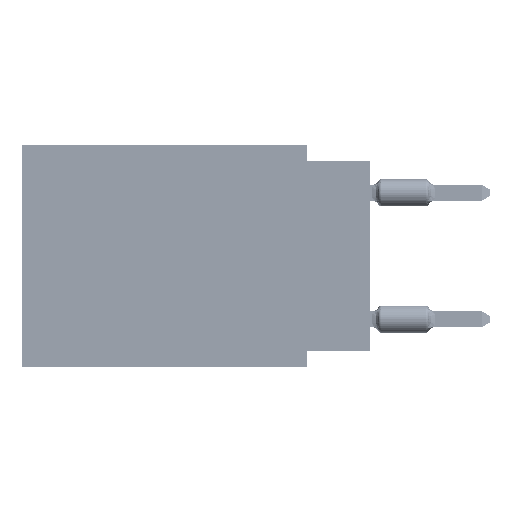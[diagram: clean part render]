
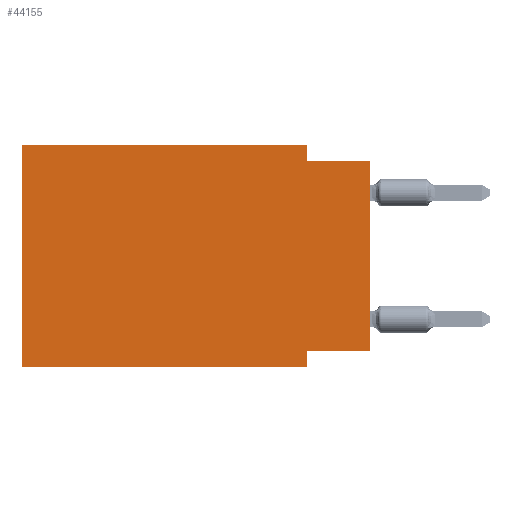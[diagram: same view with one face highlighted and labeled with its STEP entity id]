
A CAD part, left-side view. The second image highlights one B-rep face of the part: STEP entity #44155.
In plain terms, the highlighted planar face has unit normal (-1, 0, 0).
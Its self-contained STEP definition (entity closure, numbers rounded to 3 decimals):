
#339 = DIRECTION ( 'NONE',  ( 0., 0., 1. ) ) ;
#1045 = VECTOR ( 'NONE', #78806, 1000. ) ;
#1608 = CARTESIAN_POINT ( 'NONE',  ( 0., 0., -0.635 ) ) ;
#4545 = EDGE_CURVE ( 'NONE', #62421, #34760, #31598, .T. ) ;
#9363 = VERTEX_POINT ( 'NONE', #24462 ) ;
#10280 = CARTESIAN_POINT ( 'NONE',  ( 0., 13.97, 0. ) ) ;
#11450 = CARTESIAN_POINT ( 'NONE',  ( 0., 2.54, -8.255 ) ) ;
#14645 = EDGE_CURVE ( 'NONE', #9363, #31797, #24974, .T. ) ;
#15021 = CARTESIAN_POINT ( 'NONE',  ( 0., 0., 0. ) ) ;
#16466 = DIRECTION ( 'NONE',  ( 0., 0., -1. ) ) ;
#16555 = DIRECTION ( 'NONE',  ( 0., 0., -1. ) ) ;
#16689 = VECTOR ( 'NONE', #16466, 1000. ) ;
#17464 = PLANE ( 'NONE',  #34880 ) ;
#17490 = VERTEX_POINT ( 'NONE', #1608 ) ;
#18042 = LINE ( 'NONE', #81406, #1045 ) ;
#20534 = ORIENTED_EDGE ( 'NONE', *, *, #48890, .T. ) ;
#22259 = LINE ( 'NONE', #86538, #33979 ) ;
#22515 = LINE ( 'NONE', #44086, #33355 ) ;
#23358 = CARTESIAN_POINT ( 'NONE',  ( 0., 2.54, 0. ) ) ;
#23904 = FACE_OUTER_BOUND ( 'NONE', #74690, .T. ) ;
#24462 = CARTESIAN_POINT ( 'NONE',  ( 0., 13.97, -8.89 ) ) ;
#24974 = LINE ( 'NONE', #10280, #47477 ) ;
#25876 = DIRECTION ( 'NONE',  ( 0., 0., 1. ) ) ;
#25960 = EDGE_CURVE ( 'NONE', #31797, #62421, #22259, .T. ) ;
#26958 = CARTESIAN_POINT ( 'NONE',  ( 0., 2.54, -0.635 ) ) ;
#28956 = DIRECTION ( 'NONE',  ( 0., 0., -1. ) ) ;
#30323 = LINE ( 'NONE', #43164, #81911 ) ;
#30335 = ORIENTED_EDGE ( 'NONE', *, *, #25960, .F. ) ;
#30776 = DIRECTION ( 'NONE',  ( 0., -1., 0. ) ) ;
#31598 = LINE ( 'NONE', #23358, #16689 ) ;
#31597 = CARTESIAN_POINT ( 'NONE',  ( 0., 0., -0.635 ) ) ;
#31797 = VERTEX_POINT ( 'NONE', #78074 ) ;
#33355 = VECTOR ( 'NONE', #28956, 1000. ) ;
#33979 = VECTOR ( 'NONE', #71390, 1000. ) ;
#34760 = VERTEX_POINT ( 'NONE', #26958 ) ;
#34880 = AXIS2_PLACEMENT_3D ( 'NONE', #59230, #87263, #16555 ) ;
#38481 = LINE ( 'NONE', #31597, #69813 ) ;
#39219 = ORIENTED_EDGE ( 'NONE', *, *, #4545, .F. ) ;
#40088 = CARTESIAN_POINT ( 'NONE',  ( 0., 2.54, 0. ) ) ;
#41419 = EDGE_CURVE ( 'NONE', #69312, #64354, #18042, .T. ) ;
#42133 = ORIENTED_EDGE ( 'NONE', *, *, #61796, .T. ) ;
#43164 = CARTESIAN_POINT ( 'NONE',  ( 0., 13.97, -8.89 ) ) ;
#44086 = CARTESIAN_POINT ( 'NONE',  ( 0., 2.54, -8.89 ) ) ;
#44155 = ADVANCED_FACE ( 'NONE', ( #23904 ), #17464, .F. ) ;
#44665 = VECTOR ( 'NONE', #339, 1000. ) ;
#47477 = VECTOR ( 'NONE', #25876, 1000. ) ;
#48513 = CARTESIAN_POINT ( 'NONE',  ( 0., 0., -8.255 ) ) ;
#48890 = EDGE_CURVE ( 'NONE', #69312, #17490, #56803, .T. ) ;
#56620 = ORIENTED_EDGE ( 'NONE', *, *, #41419, .F. ) ;
#56803 = LINE ( 'NONE', #15021, #44665 ) ;
#56969 = ORIENTED_EDGE ( 'NONE', *, *, #86763, .F. ) ;
#59230 = CARTESIAN_POINT ( 'NONE',  ( 0., 13.97, 0. ) ) ;
#61796 = EDGE_CURVE ( 'NONE', #9363, #90607, #30323, .T. ) ;
#62421 = VERTEX_POINT ( 'NONE', #40088 ) ;
#64354 = VERTEX_POINT ( 'NONE', #11450 ) ;
#69312 = VERTEX_POINT ( 'NONE', #48513 ) ;
#69813 = VECTOR ( 'NONE', #87619, 1000. ) ;
#71271 = CARTESIAN_POINT ( 'NONE',  ( 0., 2.54, -8.89 ) ) ;
#71390 = DIRECTION ( 'NONE',  ( 0., -1., 0. ) ) ;
#71917 = ORIENTED_EDGE ( 'NONE', *, *, #84685, .F. ) ;
#74690 = EDGE_LOOP ( 'NONE', ( #20534, #71917, #39219, #30335, #83696, #42133, #56969, #56620 ) ) ;
#78074 = CARTESIAN_POINT ( 'NONE',  ( 0., 13.97, 0. ) ) ;
#78806 = DIRECTION ( 'NONE',  ( 0., 1., 0. ) ) ;
#81406 = CARTESIAN_POINT ( 'NONE',  ( 0., 0., -8.255 ) ) ;
#81911 = VECTOR ( 'NONE', #30776, 1000. ) ;
#83696 = ORIENTED_EDGE ( 'NONE', *, *, #14645, .F. ) ;
#84685 = EDGE_CURVE ( 'NONE', #34760, #17490, #38481, .T. ) ;
#86538 = CARTESIAN_POINT ( 'NONE',  ( 0., 13.97, 0. ) ) ;
#86763 = EDGE_CURVE ( 'NONE', #64354, #90607, #22515, .T. ) ;
#87263 = DIRECTION ( 'NONE',  ( 1., 0., 0. ) ) ;
#87619 = DIRECTION ( 'NONE',  ( 0., -1., 0. ) ) ;
#90607 = VERTEX_POINT ( 'NONE', #71271 ) ;
